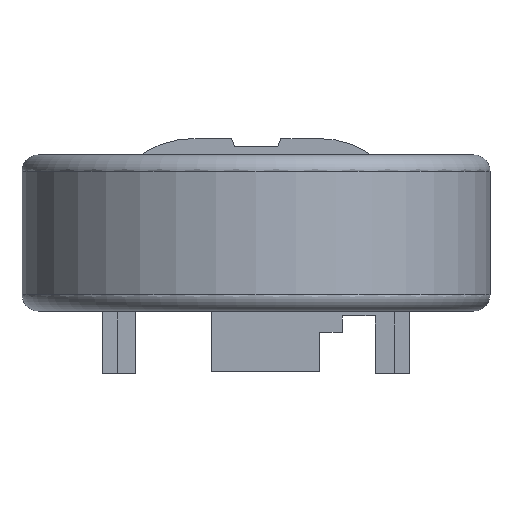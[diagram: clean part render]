
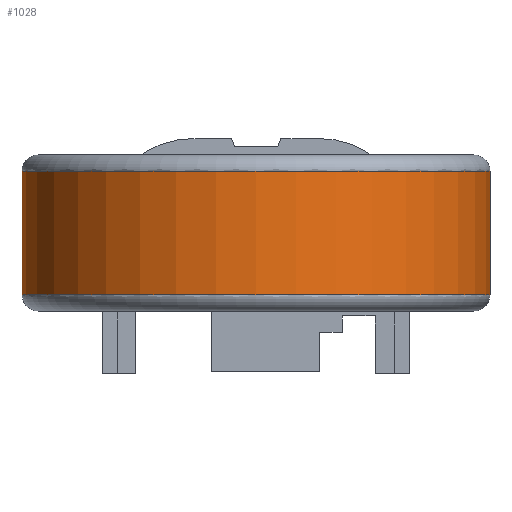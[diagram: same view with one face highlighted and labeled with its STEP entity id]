
A CAD part, left-side view. The second image highlights one B-rep face of the part: STEP entity #1028.
In plain terms, the highlighted cylindrical face has radius 14.25 mm (diameter 28.5 mm), a partial arc.
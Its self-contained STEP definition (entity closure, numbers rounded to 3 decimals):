
#76=FACE_OUTER_BOUND('',#134,.T.);
#134=EDGE_LOOP('',(#751,#752,#753,#754));
#193=LINE('',#1510,#304);
#204=LINE('',#1579,#315);
#304=VECTOR('',#1195,10.);
#315=VECTOR('',#1230,10.);
#421=CIRCLE('',#1111,14.25);
#423=CIRCLE('',#1114,14.25);
#444=VERTEX_POINT('',#1487);
#447=VERTEX_POINT('',#1508);
#464=VERTEX_POINT('',#1561);
#465=VERTEX_POINT('',#1578);
#548=EDGE_CURVE('',#447,#444,#193,.T.);
#569=EDGE_CURVE('',#464,#465,#204,.T.);
#581=EDGE_CURVE('',#444,#464,#421,.T.);
#583=EDGE_CURVE('',#465,#447,#423,.T.);
#751=ORIENTED_EDGE('',*,*,#581,.F.);
#752=ORIENTED_EDGE('',*,*,#548,.F.);
#753=ORIENTED_EDGE('',*,*,#583,.F.);
#754=ORIENTED_EDGE('',*,*,#569,.F.);
#1008=CYLINDRICAL_SURFACE('',#1113,14.25);
#1028=ADVANCED_FACE('',(#76),#1008,.T.);
#1111=AXIS2_PLACEMENT_3D('',#1614,#1250,#1251);
#1113=AXIS2_PLACEMENT_3D('',#1616,#1254,#1255);
#1114=AXIS2_PLACEMENT_3D('',#1617,#1256,#1257);
#1195=DIRECTION('',(0.,0.,1.));
#1230=DIRECTION('',(0.,0.,-1.));
#1250=DIRECTION('center_axis',(0.,0.,
1.));
#1251=DIRECTION('ref_axis',(-1.,0.,0.));
#1254=DIRECTION('center_axis',(0.,0.,-1.));
#1255=DIRECTION('ref_axis',(-1.,0.,0.));
#1256=DIRECTION('center_axis',(0.,0.,
-1.));
#1257=DIRECTION('ref_axis',(-1.,0.,0.));
#1487=CARTESIAN_POINT('',(-77.503,82.681,24.411));
#1508=CARTESIAN_POINT('',(-77.503,82.681,16.909));
#1510=CARTESIAN_POINT('',(-77.503,82.681,25.411));
#1561=CARTESIAN_POINT('',(-77.503,64.008,24.411));
#1578=CARTESIAN_POINT('',(-77.503,64.008,16.909));
#1579=CARTESIAN_POINT('',(-77.503,64.008,25.411));
#1614=CARTESIAN_POINT('Origin',(-88.268,73.344,24.411));
#1616=CARTESIAN_POINT('Origin',(-88.268,73.344,25.411));
#1617=CARTESIAN_POINT('Origin',(-88.268,73.344,16.909));
